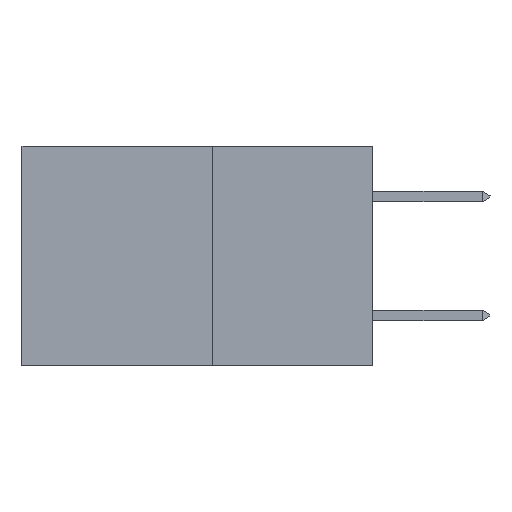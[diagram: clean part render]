
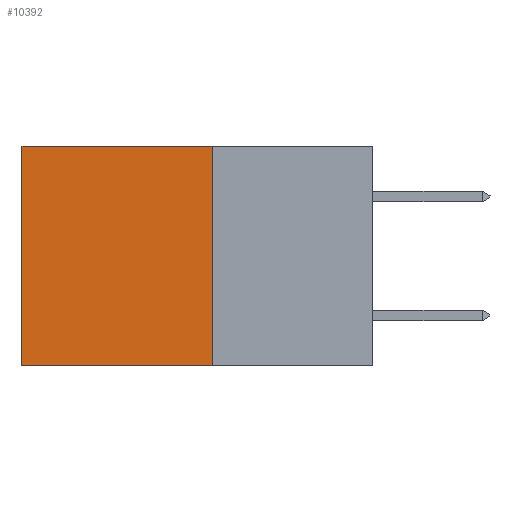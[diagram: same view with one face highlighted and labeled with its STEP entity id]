
A CAD part, left-side view. The second image highlights one B-rep face of the part: STEP entity #10392.
In plain terms, the highlighted planar face has unit normal (-1, 0, 0).
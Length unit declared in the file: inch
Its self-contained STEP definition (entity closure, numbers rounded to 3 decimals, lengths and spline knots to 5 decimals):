
#1 = DIRECTION ( 'NONE',  ( 0., 0., -1. ) ) ;
#46 = DIRECTION ( 'NONE',  ( 0., 0., -1. ) ) ;
#319 = VERTEX_POINT ( 'NONE', #5072 ) ;
#431 = VERTEX_POINT ( 'NONE', #9963 ) ;
#484 = ORIENTED_EDGE ( 'NONE', *, *, #3593, .F. ) ;
#862 = EDGE_CURVE ( 'NONE', #2727, #3679, #17048, .T. ) ;
#1295 = LINE ( 'NONE', #4434, #9237 ) ;
#1346 = AXIS2_PLACEMENT_3D ( 'NONE', #14156, #14166, #1 ) ;
#2208 = EDGE_LOOP ( 'NONE', ( #7207, #484, #3474, #14158 ) ) ;
#2639 = LINE ( 'NONE', #11664, #6362 ) ;
#2727 = VERTEX_POINT ( 'NONE', #11232 ) ;
#3148 = LINE ( 'NONE', #13942, #18113 ) ;
#3474 = ORIENTED_EDGE ( 'NONE', *, *, #862, .F. ) ;
#3593 = EDGE_CURVE ( 'NONE', #3679, #431, #3148, .T. ) ;
#3679 = VERTEX_POINT ( 'NONE', #11208 ) ;
#4434 = CARTESIAN_POINT ( 'NONE',  ( 0.277, 0.27, 0. ) ) ;
#5072 = CARTESIAN_POINT ( 'NONE',  ( 0.277, 0.59, 0. ) ) ;
#6212 = EDGE_CURVE ( 'NONE', #319, #431, #2639, .T. ) ;
#6362 = VECTOR ( 'NONE', #11645, 39.37008 ) ;
#7207 = ORIENTED_EDGE ( 'NONE', *, *, #6212, .T. ) ;
#7662 = EDGE_CURVE ( 'NONE', #2727, #319, #1295, .T. ) ;
#9237 = VECTOR ( 'NONE', #16996, 39.37008 ) ;
#9963 = CARTESIAN_POINT ( 'NONE',  ( 0.277, 0.59, -0.37 ) ) ;
#10392 = ADVANCED_FACE ( 'NONE', ( #18846 ), #18340, .F. ) ;
#11208 = CARTESIAN_POINT ( 'NONE',  ( 0.277, 0.27, -0.37 ) ) ;
#11232 = CARTESIAN_POINT ( 'NONE',  ( 0.277, 0.27, 0. ) ) ;
#11645 = DIRECTION ( 'NONE',  ( 0., 0., -1. ) ) ;
#11664 = CARTESIAN_POINT ( 'NONE',  ( 0.277, 0.59, -0.37 ) ) ;
#13201 = VECTOR ( 'NONE', #46, 39.37008 ) ;
#13912 = DIRECTION ( 'NONE',  ( 0., 1., 0. ) ) ;
#13942 = CARTESIAN_POINT ( 'NONE',  ( 0.277, 0.27, -0.37 ) ) ;
#14156 = CARTESIAN_POINT ( 'NONE',  ( 0.277, 0.27, -0.37 ) ) ;
#14158 = ORIENTED_EDGE ( 'NONE', *, *, #7662, .T. ) ;
#14166 = DIRECTION ( 'NONE',  ( 1., 0., 0. ) ) ;
#16996 = DIRECTION ( 'NONE',  ( 0., 1., 0. ) ) ;
#17048 = LINE ( 'NONE', #17510, #13201 ) ;
#17510 = CARTESIAN_POINT ( 'NONE',  ( 0.277, 0.27, -0.37 ) ) ;
#18113 = VECTOR ( 'NONE', #13912, 39.37008 ) ;
#18340 = PLANE ( 'NONE',  #1346 ) ;
#18846 = FACE_OUTER_BOUND ( 'NONE', #2208, .T. ) ;
